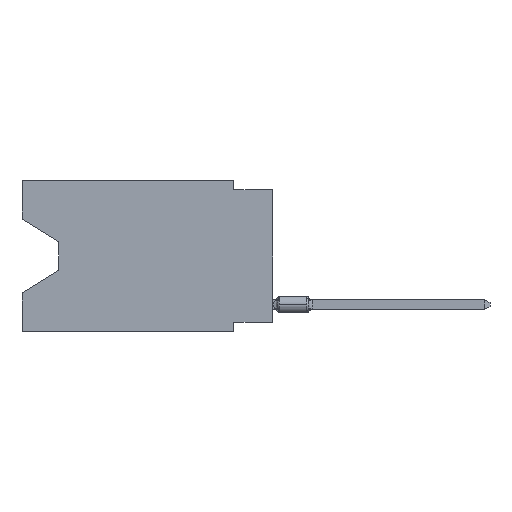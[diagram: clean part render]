
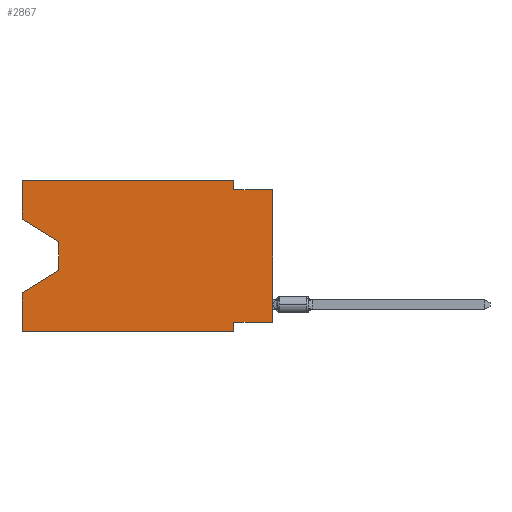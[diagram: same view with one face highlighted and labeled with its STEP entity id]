
A CAD part, left-side view. The second image highlights one B-rep face of the part: STEP entity #2867.
In plain terms, the highlighted planar face has unit normal (-1, 0, 0).
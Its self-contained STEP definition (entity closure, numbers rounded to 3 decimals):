
#58 = VECTOR ( 'NONE', #8331, 1000. ) ;
#150 = CARTESIAN_POINT ( 'NONE',  ( 0., 16.383, 0. ) ) ;
#228 = CARTESIAN_POINT ( 'NONE',  ( 0., 16.383, -2.546 ) ) ;
#359 = PLANE ( 'NONE',  #18396 ) ;
#562 = CARTESIAN_POINT ( 'NONE',  ( 0., 13.97, -5.893 ) ) ;
#807 = EDGE_CURVE ( 'NONE', #9981, #14348, #8075, .T. ) ;
#1172 = CARTESIAN_POINT ( 'NONE',  ( 0., 2.54, 0. ) ) ;
#1315 = VERTEX_POINT ( 'NONE', #17943 ) ;
#1585 = EDGE_CURVE ( 'NONE', #21978, #2475, #5374, .T. ) ;
#1881 = DIRECTION ( 'NONE',  ( 0., 0., 1. ) ) ;
#2026 = ORIENTED_EDGE ( 'NONE', *, *, #9017, .F. ) ;
#2285 = CARTESIAN_POINT ( 'NONE',  ( 0., 0., -9.271 ) ) ;
#2399 = VERTEX_POINT ( 'NONE', #150 ) ;
#2475 = VERTEX_POINT ( 'NONE', #11597 ) ;
#2628 = EDGE_CURVE ( 'NONE', #20169, #13322, #18436, .T. ) ;
#2739 = CARTESIAN_POINT ( 'NONE',  ( 0., 16.383, -9.906 ) ) ;
#2830 = VECTOR ( 'NONE', #15309, 1000. ) ;
#2867 = ADVANCED_FACE ( 'NONE', ( #17766 ), #359, .F. ) ;
#3812 = EDGE_CURVE ( 'NONE', #15313, #1315, #11382, .T. ) ;
#3915 = CARTESIAN_POINT ( 'NONE',  ( 0., 13.97, -4.013 ) ) ;
#3938 = LINE ( 'NONE', #2285, #18637 ) ;
#3960 = VERTEX_POINT ( 'NONE', #2739 ) ;
#4456 = DIRECTION ( 'NONE',  ( 0., -1., 0. ) ) ;
#4487 = CARTESIAN_POINT ( 'NONE',  ( 0., 2.54, -0.635 ) ) ;
#4576 = CARTESIAN_POINT ( 'NONE',  ( 0., 16.383, 0. ) ) ;
#4698 = ORIENTED_EDGE ( 'NONE', *, *, #1585, .T. ) ;
#5049 = CARTESIAN_POINT ( 'NONE',  ( 0., 0., -0.635 ) ) ;
#5067 = CARTESIAN_POINT ( 'NONE',  ( 0., 2.54, -9.906 ) ) ;
#5374 = LINE ( 'NONE', #19078, #20351 ) ;
#5562 = CARTESIAN_POINT ( 'NONE',  ( 0., 0., -9.271 ) ) ;
#6057 = LINE ( 'NONE', #19286, #12910 ) ;
#6221 = DIRECTION ( 'NONE',  ( 0., 0., -1. ) ) ;
#6842 = LINE ( 'NONE', #4576, #10122 ) ;
#7100 = LINE ( 'NONE', #5067, #20379 ) ;
#7160 = CARTESIAN_POINT ( 'NONE',  ( 0., 16.383, -9.906 ) ) ;
#7471 = EDGE_CURVE ( 'NONE', #13322, #1315, #10885, .T. ) ;
#7587 = CARTESIAN_POINT ( 'NONE',  ( 0., 0., 0. ) ) ;
#7665 = EDGE_CURVE ( 'NONE', #21978, #2399, #6057, .T. ) ;
#7685 = EDGE_CURVE ( 'NONE', #2475, #9981, #9889, .T. ) ;
#7888 = CARTESIAN_POINT ( 'NONE',  ( 0., 16.383, 0. ) ) ;
#8075 = LINE ( 'NONE', #562, #58 ) ;
#8331 = DIRECTION ( 'NONE',  ( 0., 0.855, -0.519 ) ) ;
#8424 = ORIENTED_EDGE ( 'NONE', *, *, #2628, .F. ) ;
#8472 = EDGE_LOOP ( 'NONE', ( #4698, #17813, #25096, #16790, #9227, #13212, #2026, #14438, #24184, #8424, #11733, #18347 ) ) ;
#9017 = EDGE_CURVE ( 'NONE', #15313, #19999, #3938, .T. ) ;
#9178 = EDGE_CURVE ( 'NONE', #3960, #14348, #6842, .T. ) ;
#9227 = ORIENTED_EDGE ( 'NONE', *, *, #11003, .T. ) ;
#9889 = LINE ( 'NONE', #3915, #11744 ) ;
#9981 = VERTEX_POINT ( 'NONE', #16498 ) ;
#10122 = VECTOR ( 'NONE', #12696, 1000. ) ;
#10885 = LINE ( 'NONE', #5049, #12942 ) ;
#11003 = EDGE_CURVE ( 'NONE', #3960, #15199, #17436, .T. ) ;
#11382 = LINE ( 'NONE', #7587, #2830 ) ;
#11597 = CARTESIAN_POINT ( 'NONE',  ( 0., 13.97, -4.013 ) ) ;
#11733 = ORIENTED_EDGE ( 'NONE', *, *, #18161, .F. ) ;
#11744 = VECTOR ( 'NONE', #11904, 1000. ) ;
#11904 = DIRECTION ( 'NONE',  ( 0., 0., -1. ) ) ;
#12294 = VECTOR ( 'NONE', #18308, 1000. ) ;
#12696 = DIRECTION ( 'NONE',  ( 0., 0., 1. ) ) ;
#12910 = VECTOR ( 'NONE', #1881, 1000. ) ;
#12942 = VECTOR ( 'NONE', #24366, 1000. ) ;
#13212 = ORIENTED_EDGE ( 'NONE', *, *, #22351, .F. ) ;
#13322 = VERTEX_POINT ( 'NONE', #4487 ) ;
#13865 = CARTESIAN_POINT ( 'NONE',  ( 0., 16.383, 0. ) ) ;
#14348 = VERTEX_POINT ( 'NONE', #16100 ) ;
#14438 = ORIENTED_EDGE ( 'NONE', *, *, #3812, .T. ) ;
#15199 = VERTEX_POINT ( 'NONE', #19576 ) ;
#15309 = DIRECTION ( 'NONE',  ( 0., 0., 1. ) ) ;
#15313 = VERTEX_POINT ( 'NONE', #5562 ) ;
#15863 = DIRECTION ( 'NONE',  ( 1., 0., 0. ) ) ;
#16100 = CARTESIAN_POINT ( 'NONE',  ( 0., 16.383, -7.36 ) ) ;
#16498 = CARTESIAN_POINT ( 'NONE',  ( 0., 13.97, -5.893 ) ) ;
#16790 = ORIENTED_EDGE ( 'NONE', *, *, #9178, .F. ) ;
#17004 = DIRECTION ( 'NONE',  ( 0., 0., -1. ) ) ;
#17436 = LINE ( 'NONE', #7160, #18714 ) ;
#17766 = FACE_OUTER_BOUND ( 'NONE', #8472, .T. ) ;
#17813 = ORIENTED_EDGE ( 'NONE', *, *, #7685, .T. ) ;
#17943 = CARTESIAN_POINT ( 'NONE',  ( 0., 0., -0.635 ) ) ;
#18026 = DIRECTION ( 'NONE',  ( 0., 1., 0. ) ) ;
#18161 = EDGE_CURVE ( 'NONE', #2399, #20169, #19579, .T. ) ;
#18308 = DIRECTION ( 'NONE',  ( 0., 0., -1. ) ) ;
#18347 = ORIENTED_EDGE ( 'NONE', *, *, #7665, .F. ) ;
#18396 = AXIS2_PLACEMENT_3D ( 'NONE', #7888, #15863, #6221 ) ;
#18436 = LINE ( 'NONE', #24052, #12294 ) ;
#18637 = VECTOR ( 'NONE', #18026, 1000. ) ;
#18714 = VECTOR ( 'NONE', #18852, 1000. ) ;
#18852 = DIRECTION ( 'NONE',  ( 0., -1., 0. ) ) ;
#19078 = CARTESIAN_POINT ( 'NONE',  ( 0., 16.383, -2.546 ) ) ;
#19286 = CARTESIAN_POINT ( 'NONE',  ( 0., 16.383, 0. ) ) ;
#19576 = CARTESIAN_POINT ( 'NONE',  ( 0., 2.54, -9.906 ) ) ;
#19579 = LINE ( 'NONE', #13865, #21188 ) ;
#19999 = VERTEX_POINT ( 'NONE', #22977 ) ;
#20169 = VERTEX_POINT ( 'NONE', #1172 ) ;
#20351 = VECTOR ( 'NONE', #24941, 1000. ) ;
#20379 = VECTOR ( 'NONE', #17004, 1000. ) ;
#21188 = VECTOR ( 'NONE', #4456, 1000. ) ;
#21978 = VERTEX_POINT ( 'NONE', #228 ) ;
#22351 = EDGE_CURVE ( 'NONE', #19999, #15199, #7100, .T. ) ;
#22977 = CARTESIAN_POINT ( 'NONE',  ( 0., 2.54, -9.271 ) ) ;
#24052 = CARTESIAN_POINT ( 'NONE',  ( 0., 2.54, 0. ) ) ;
#24184 = ORIENTED_EDGE ( 'NONE', *, *, #7471, .F. ) ;
#24366 = DIRECTION ( 'NONE',  ( 0., -1., 0. ) ) ;
#24941 = DIRECTION ( 'NONE',  ( 0., -0.855, -0.519 ) ) ;
#25096 = ORIENTED_EDGE ( 'NONE', *, *, #807, .T. ) ;
